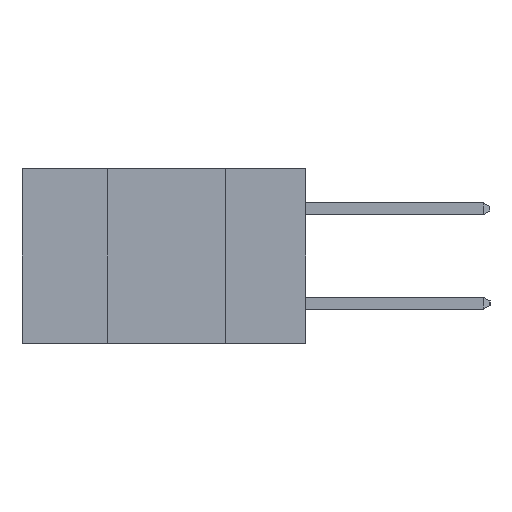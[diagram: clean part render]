
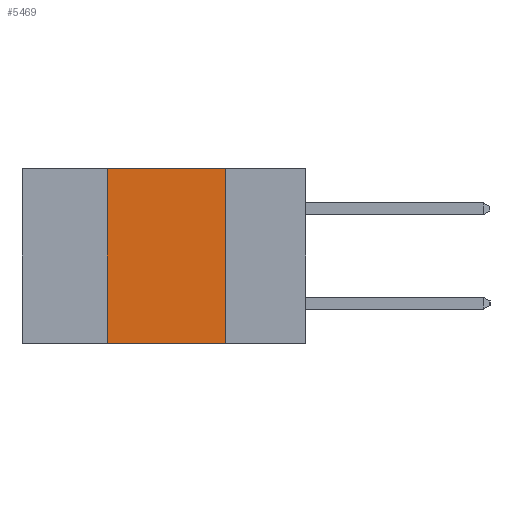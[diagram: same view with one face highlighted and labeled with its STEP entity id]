
A CAD part, left-side view. The second image highlights one B-rep face of the part: STEP entity #5469.
In plain terms, the highlighted planar face has unit normal (-1, 0, 0).
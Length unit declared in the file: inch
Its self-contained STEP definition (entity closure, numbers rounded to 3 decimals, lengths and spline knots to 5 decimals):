
#1167 = CARTESIAN_POINT ( 'NONE',  ( 0., 0.42, -0.37 ) ) ;
#1655 = DIRECTION ( 'NONE',  ( 0., -1., 0. ) ) ;
#1726 = CARTESIAN_POINT ( 'NONE',  ( 0., 0.6, -0.37 ) ) ;
#2217 = DIRECTION ( 'NONE',  ( 0., 0., -1. ) ) ;
#2237 = DIRECTION ( 'NONE',  ( 1., 0., 0. ) ) ;
#2254 = CARTESIAN_POINT ( 'NONE',  ( 0., 0.6, 0. ) ) ;
#2317 = PLANE ( 'NONE',  #8503 ) ;
#2448 = CARTESIAN_POINT ( 'NONE',  ( 0., 0.42, -0.37 ) ) ;
#4076 = ORIENTED_EDGE ( 'NONE', *, *, #11738, .T. ) ;
#4086 = CARTESIAN_POINT ( 'NONE',  ( 0., 0.17, 0. ) ) ;
#4223 = ORIENTED_EDGE ( 'NONE', *, *, #15503, .F. ) ;
#4548 = CARTESIAN_POINT ( 'NONE',  ( 0., 0.6, 0. ) ) ;
#5461 = VERTEX_POINT ( 'NONE', #2448 ) ;
#5469 = ADVANCED_FACE ( 'NONE', ( #6156 ), #2317, .F. ) ;
#6156 = FACE_OUTER_BOUND ( 'NONE', #8989, .T. ) ;
#6159 = VECTOR ( 'NONE', #6884, 39.37008 ) ;
#6438 = LINE ( 'NONE', #4548, #17399 ) ;
#6604 = LINE ( 'NONE', #14060, #6159 ) ;
#6884 = DIRECTION ( 'NONE',  ( 0., 0., -1. ) ) ;
#7332 = VERTEX_POINT ( 'NONE', #11768 ) ;
#8503 = AXIS2_PLACEMENT_3D ( 'NONE', #2254, #2237, #2217 ) ;
#8989 = EDGE_LOOP ( 'NONE', ( #17345, #4223, #12808, #4076 ) ) ;
#9566 = LINE ( 'NONE', #1167, #12952 ) ;
#10111 = DIRECTION ( 'NONE',  ( 0., 0., 1. ) ) ;
#10383 = LINE ( 'NONE', #1726, #14176 ) ;
#11738 = EDGE_CURVE ( 'NONE', #5461, #17509, #10383, .T. ) ;
#11757 = CARTESIAN_POINT ( 'NONE',  ( 0., 0.17, -0.37 ) ) ;
#11768 = CARTESIAN_POINT ( 'NONE',  ( 0., 0.42, 0. ) ) ;
#12808 = ORIENTED_EDGE ( 'NONE', *, *, #17422, .F. ) ;
#12952 = VECTOR ( 'NONE', #10111, 39.37008 ) ;
#13270 = DIRECTION ( 'NONE',  ( 0., -1., 0. ) ) ;
#14060 = CARTESIAN_POINT ( 'NONE',  ( 0., 0.17, -0.37 ) ) ;
#14176 = VECTOR ( 'NONE', #1655, 39.37008 ) ;
#15503 = EDGE_CURVE ( 'NONE', #7332, #17332, #6438, .T. ) ;
#16664 = EDGE_CURVE ( 'NONE', #17332, #17509, #6604, .T. ) ;
#17332 = VERTEX_POINT ( 'NONE', #4086 ) ;
#17345 = ORIENTED_EDGE ( 'NONE', *, *, #16664, .F. ) ;
#17399 = VECTOR ( 'NONE', #13270, 39.37008 ) ;
#17422 = EDGE_CURVE ( 'NONE', #5461, #7332, #9566, .T. ) ;
#17509 = VERTEX_POINT ( 'NONE', #11757 ) ;
